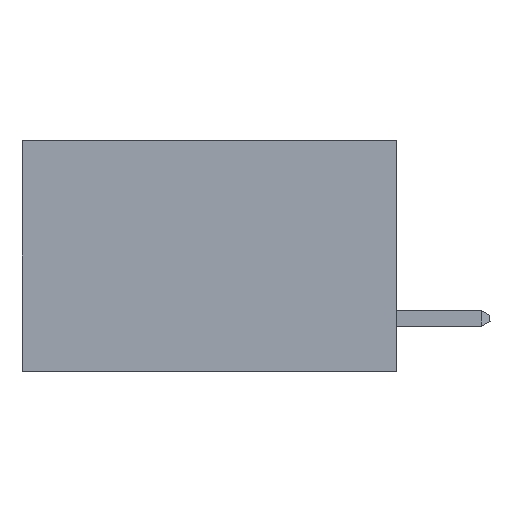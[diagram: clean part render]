
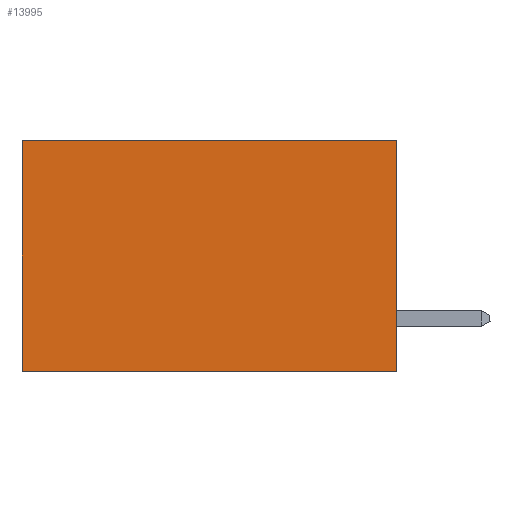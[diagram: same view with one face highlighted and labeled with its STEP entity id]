
A CAD part, left-side view. The second image highlights one B-rep face of the part: STEP entity #13995.
In plain terms, the highlighted planar face has unit normal (-1, 0, 0).
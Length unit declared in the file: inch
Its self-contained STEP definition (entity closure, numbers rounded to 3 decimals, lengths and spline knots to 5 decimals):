
#388 = CARTESIAN_POINT ( 'NONE',  ( 0.298, 0.6, 0. ) ) ;
#990 = DIRECTION ( 'NONE',  ( 0., 1., 0. ) ) ;
#1374 = VERTEX_POINT ( 'NONE', #388 ) ;
#1745 = DIRECTION ( 'NONE',  ( 0., 1., 0. ) ) ;
#2168 = ORIENTED_EDGE ( 'NONE', *, *, #7870, .F. ) ;
#3138 = DIRECTION ( 'NONE',  ( 0., 0., -1. ) ) ;
#3352 = VECTOR ( 'NONE', #990, 39.37008 ) ;
#3654 = VECTOR ( 'NONE', #10833, 39.37008 ) ;
#3859 = EDGE_CURVE ( 'NONE', #13233, #4809, #13223, .T. ) ;
#4809 = VERTEX_POINT ( 'NONE', #12186 ) ;
#5212 = VECTOR ( 'NONE', #3138, 39.37008 ) ;
#6216 = CARTESIAN_POINT ( 'NONE',  ( 0.298, 0.6, 0. ) ) ;
#6313 = EDGE_CURVE ( 'NONE', #1374, #11253, #7559, .T. ) ;
#6879 = CARTESIAN_POINT ( 'NONE',  ( 0.298, 0., 0. ) ) ;
#7559 = LINE ( 'NONE', #6216, #5212 ) ;
#7630 = CARTESIAN_POINT ( 'NONE',  ( 0.298, 0., 0. ) ) ;
#7870 = EDGE_CURVE ( 'NONE', #4809, #11253, #8400, .T. ) ;
#8086 = LINE ( 'NONE', #13155, #9151 ) ;
#8196 = CARTESIAN_POINT ( 'NONE',  ( 0.298, 0., 0. ) ) ;
#8400 = LINE ( 'NONE', #10060, #3352 ) ;
#8630 = PLANE ( 'NONE',  #10877 ) ;
#9076 = ORIENTED_EDGE ( 'NONE', *, *, #3859, .F. ) ;
#9151 = VECTOR ( 'NONE', #1745, 39.37008 ) ;
#9784 = DIRECTION ( 'NONE',  ( 1., 0., 0. ) ) ;
#10060 = CARTESIAN_POINT ( 'NONE',  ( 0.298, 0., -0.37 ) ) ;
#10833 = DIRECTION ( 'NONE',  ( 0., 0., -1. ) ) ;
#10877 = AXIS2_PLACEMENT_3D ( 'NONE', #7630, #9784, #12297 ) ;
#10978 = EDGE_CURVE ( 'NONE', #13233, #1374, #8086, .T. ) ;
#11231 = FACE_OUTER_BOUND ( 'NONE', #12222, .T. ) ;
#11253 = VERTEX_POINT ( 'NONE', #11606 ) ;
#11606 = CARTESIAN_POINT ( 'NONE',  ( 0.298, 0.6, -0.37 ) ) ;
#12186 = CARTESIAN_POINT ( 'NONE',  ( 0.298, 0., -0.37 ) ) ;
#12222 = EDGE_LOOP ( 'NONE', ( #13479, #2168, #9076, #13100 ) ) ;
#12297 = DIRECTION ( 'NONE',  ( 0., 0., -1. ) ) ;
#13100 = ORIENTED_EDGE ( 'NONE', *, *, #10978, .T. ) ;
#13155 = CARTESIAN_POINT ( 'NONE',  ( 0.298, 0., 0. ) ) ;
#13223 = LINE ( 'NONE', #8196, #3654 ) ;
#13233 = VERTEX_POINT ( 'NONE', #6879 ) ;
#13479 = ORIENTED_EDGE ( 'NONE', *, *, #6313, .T. ) ;
#13995 = ADVANCED_FACE ( 'NONE', ( #11231 ), #8630, .F. ) ;
